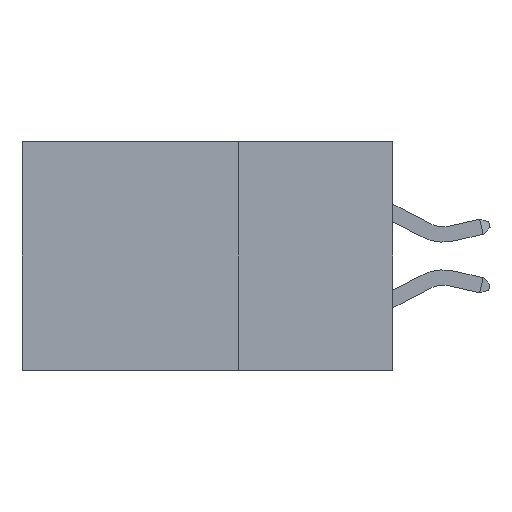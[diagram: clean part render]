
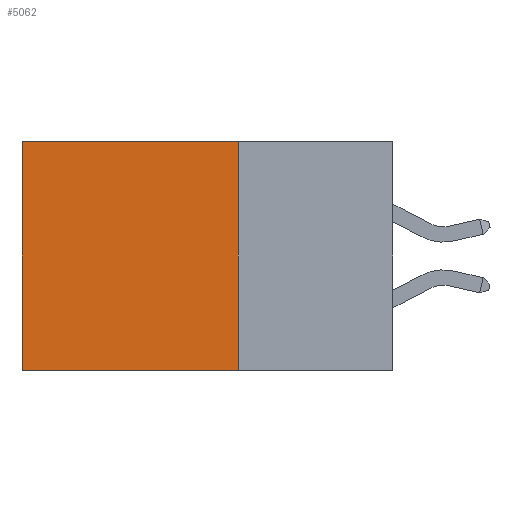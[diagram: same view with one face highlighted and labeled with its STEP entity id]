
A CAD part, left-side view. The second image highlights one B-rep face of the part: STEP entity #5062.
In plain terms, the highlighted planar face has unit normal (-1, 0, 0).
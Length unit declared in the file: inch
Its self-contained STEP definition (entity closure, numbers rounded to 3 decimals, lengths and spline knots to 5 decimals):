
#66 = VERTEX_POINT ( 'NONE', #1023 ) ;
#188 = CARTESIAN_POINT ( 'NONE',  ( 0.2875, 0.6, 0. ) ) ;
#373 = EDGE_CURVE ( 'NONE', #3820, #3790, #2705, .T. ) ;
#462 = VECTOR ( 'NONE', #9865, 39.37008 ) ;
#836 = CARTESIAN_POINT ( 'NONE',  ( 0.2875, 0.25, 0. ) ) ;
#1023 = CARTESIAN_POINT ( 'NONE',  ( 0.2875, 0.6, -0.37 ) ) ;
#1402 = ORIENTED_EDGE ( 'NONE', *, *, #3544, .T. ) ;
#2150 = CARTESIAN_POINT ( 'NONE',  ( 0.2875, 0.25, 0. ) ) ;
#2331 = ORIENTED_EDGE ( 'NONE', *, *, #3425, .F. ) ;
#2581 = CARTESIAN_POINT ( 'NONE',  ( 0.2875, 0.25, -0.37 ) ) ;
#2705 = LINE ( 'NONE', #4734, #462 ) ;
#3041 = LINE ( 'NONE', #3796, #9295 ) ;
#3380 = FACE_OUTER_BOUND ( 'NONE', #6628, .T. ) ;
#3425 = EDGE_CURVE ( 'NONE', #3790, #66, #6178, .T. ) ;
#3498 = CARTESIAN_POINT ( 'NONE',  ( 0.2875, 0.25, -0.37 ) ) ;
#3515 = DIRECTION ( 'NONE',  ( 0., 1., 0. ) ) ;
#3544 = EDGE_CURVE ( 'NONE', #7115, #66, #3041, .T. ) ;
#3599 = DIRECTION ( 'NONE',  ( 0., 0., -1. ) ) ;
#3790 = VERTEX_POINT ( 'NONE', #2581 ) ;
#3796 = CARTESIAN_POINT ( 'NONE',  ( 0.2875, 0.6, 0. ) ) ;
#3804 = DIRECTION ( 'NONE',  ( 0., 0., -1. ) ) ;
#3820 = VERTEX_POINT ( 'NONE', #2150 ) ;
#4734 = CARTESIAN_POINT ( 'NONE',  ( 0.2875, 0.25, 0. ) ) ;
#4755 = ORIENTED_EDGE ( 'NONE', *, *, #5458, .T. ) ;
#5062 = ADVANCED_FACE ( 'NONE', ( #3380 ), #7551, .F. ) ;
#5458 = EDGE_CURVE ( 'NONE', #3820, #7115, #6422, .T. ) ;
#6166 = ORIENTED_EDGE ( 'NONE', *, *, #373, .F. ) ;
#6178 = LINE ( 'NONE', #3498, #9980 ) ;
#6320 = AXIS2_PLACEMENT_3D ( 'NONE', #6713, #8341, #3599 ) ;
#6422 = LINE ( 'NONE', #836, #6661 ) ;
#6537 = DIRECTION ( 'NONE',  ( 0., 1., 0. ) ) ;
#6628 = EDGE_LOOP ( 'NONE', ( #1402, #2331, #6166, #4755 ) ) ;
#6661 = VECTOR ( 'NONE', #6537, 39.37008 ) ;
#6713 = CARTESIAN_POINT ( 'NONE',  ( 0.2875, 0.25, 0. ) ) ;
#7115 = VERTEX_POINT ( 'NONE', #188 ) ;
#7551 = PLANE ( 'NONE',  #6320 ) ;
#8341 = DIRECTION ( 'NONE',  ( 1., 0., 0. ) ) ;
#9295 = VECTOR ( 'NONE', #3804, 39.37008 ) ;
#9865 = DIRECTION ( 'NONE',  ( 0., 0., -1. ) ) ;
#9980 = VECTOR ( 'NONE', #3515, 39.37008 ) ;
